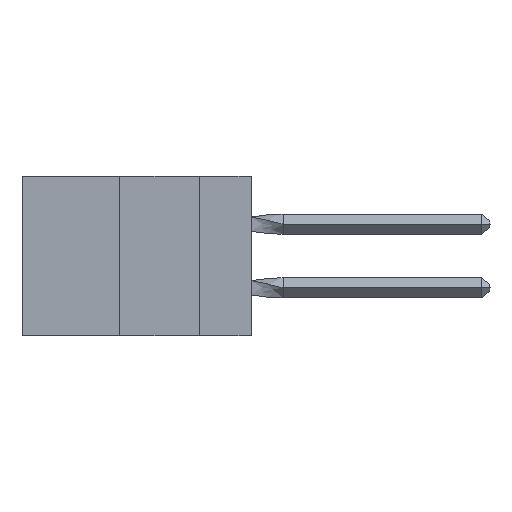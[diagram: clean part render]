
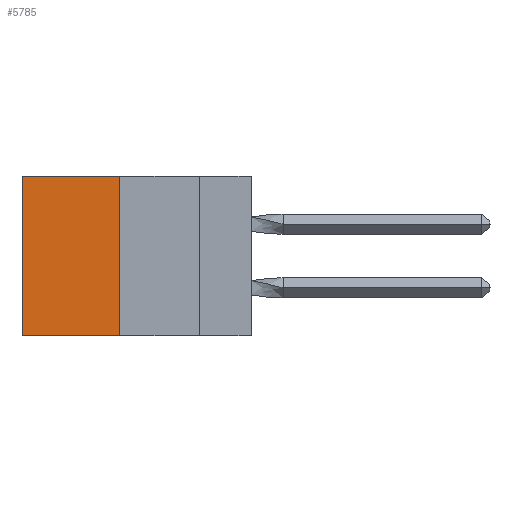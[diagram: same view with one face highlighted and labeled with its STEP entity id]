
A CAD part, left-side view. The second image highlights one B-rep face of the part: STEP entity #5785.
In plain terms, the highlighted planar face has unit normal (-1, 0, 0).
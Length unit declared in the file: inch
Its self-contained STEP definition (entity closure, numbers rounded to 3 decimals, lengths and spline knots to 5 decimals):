
#685 = DIRECTION ( 'NONE',  ( 0., 0., -1. ) ) ;
#1779 = CARTESIAN_POINT ( 'NONE',  ( 0.305, 0.413, -0.5 ) ) ;
#2476 = EDGE_CURVE ( 'NONE', #19206, #9842, #29978, .T. ) ;
#3597 = AXIS2_PLACEMENT_3D ( 'NONE', #35307, #4845, #7872 ) ;
#3645 = EDGE_LOOP ( 'NONE', ( #5895, #7513, #17646, #5788 ) ) ;
#4490 = DIRECTION ( 'NONE',  ( 0., 1., 0. ) ) ;
#4845 = DIRECTION ( 'NONE',  ( 1., 0., 0. ) ) ;
#5785 = ADVANCED_FACE ( 'NONE', ( #22358 ), #21552, .F. ) ;
#5788 = ORIENTED_EDGE ( 'NONE', *, *, #9772, .T. ) ;
#5895 = ORIENTED_EDGE ( 'NONE', *, *, #2476, .T. ) ;
#7513 = ORIENTED_EDGE ( 'NONE', *, *, #30554, .F. ) ;
#7872 = DIRECTION ( 'NONE',  ( 0., 0., -1. ) ) ;
#8519 = VERTEX_POINT ( 'NONE', #27566 ) ;
#8819 = LINE ( 'NONE', #1779, #11380 ) ;
#9523 = CARTESIAN_POINT ( 'NONE',  ( 0.305, 0.72, 0. ) ) ;
#9772 = EDGE_CURVE ( 'NONE', #8519, #19206, #16404, .T. ) ;
#9842 = VERTEX_POINT ( 'NONE', #31225 ) ;
#11380 = VECTOR ( 'NONE', #4490, 39.37008 ) ;
#11419 = CARTESIAN_POINT ( 'NONE',  ( 0.305, 0.413, 0. ) ) ;
#14299 = VECTOR ( 'NONE', #19143, 39.37008 ) ;
#16404 = LINE ( 'NONE', #11419, #14299 ) ;
#16584 = DIRECTION ( 'NONE',  ( 0., 0., -1. ) ) ;
#16841 = CARTESIAN_POINT ( 'NONE',  ( 0.305, 0.72, -0.5 ) ) ;
#17646 = ORIENTED_EDGE ( 'NONE', *, *, #35345, .F. ) ;
#19143 = DIRECTION ( 'NONE',  ( 0., 1., 0. ) ) ;
#19206 = VERTEX_POINT ( 'NONE', #9523 ) ;
#20040 = LINE ( 'NONE', #28276, #26554 ) ;
#21552 = PLANE ( 'NONE',  #3597 ) ;
#22358 = FACE_OUTER_BOUND ( 'NONE', #3645, .T. ) ;
#24555 = VERTEX_POINT ( 'NONE', #28212 ) ;
#26062 = VECTOR ( 'NONE', #16584, 39.37008 ) ;
#26554 = VECTOR ( 'NONE', #685, 39.37008 ) ;
#27566 = CARTESIAN_POINT ( 'NONE',  ( 0.305, 0.413, 0. ) ) ;
#28212 = CARTESIAN_POINT ( 'NONE',  ( 0.305, 0.413, -0.5 ) ) ;
#28276 = CARTESIAN_POINT ( 'NONE',  ( 0.305, 0.413, -0.5 ) ) ;
#29978 = LINE ( 'NONE', #16841, #26062 ) ;
#30554 = EDGE_CURVE ( 'NONE', #24555, #9842, #8819, .T. ) ;
#31225 = CARTESIAN_POINT ( 'NONE',  ( 0.305, 0.72, -0.5 ) ) ;
#35307 = CARTESIAN_POINT ( 'NONE',  ( 0.305, 0.413, -0.5 ) ) ;
#35345 = EDGE_CURVE ( 'NONE', #8519, #24555, #20040, .T. ) ;
